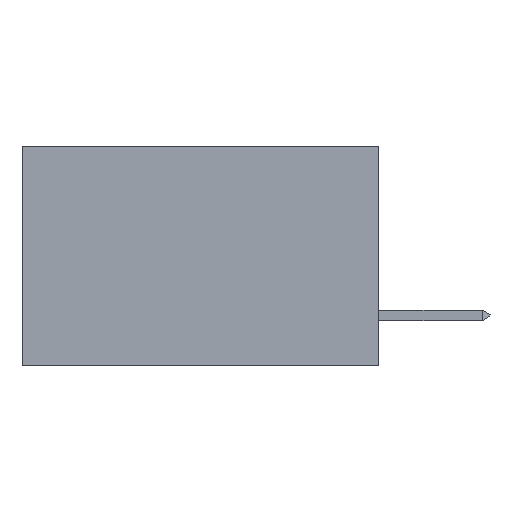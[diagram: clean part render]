
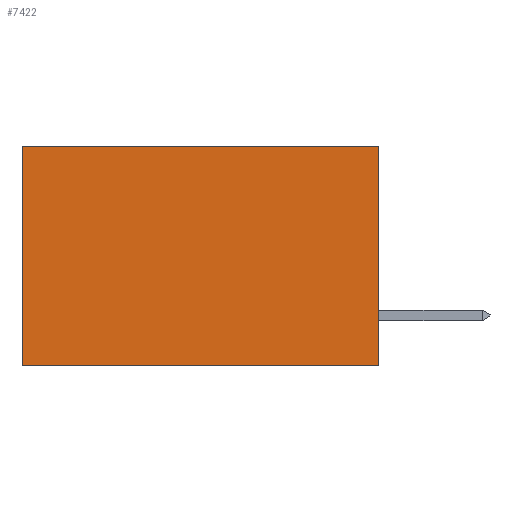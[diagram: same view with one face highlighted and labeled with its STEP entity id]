
A CAD part, left-side view. The second image highlights one B-rep face of the part: STEP entity #7422.
In plain terms, the highlighted planar face has unit normal (-1, 0, 0).
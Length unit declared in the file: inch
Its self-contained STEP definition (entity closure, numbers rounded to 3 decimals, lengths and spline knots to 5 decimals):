
#346 = EDGE_CURVE ( 'NONE', #3308, #4893, #1380, .T. ) ;
#358 = EDGE_CURVE ( 'NONE', #6321, #9454, #1969, .T. ) ;
#552 = AXIS2_PLACEMENT_3D ( 'NONE', #7037, #2612, #9248 ) ;
#845 = ORIENTED_EDGE ( 'NONE', *, *, #5354, .T. ) ;
#1380 = LINE ( 'NONE', #7633, #3596 ) ;
#1655 = DIRECTION ( 'NONE',  ( 0., 1., 0. ) ) ;
#1969 = LINE ( 'NONE', #5311, #6136 ) ;
#2228 = LINE ( 'NONE', #3424, #8669 ) ;
#2229 = CARTESIAN_POINT ( 'NONE',  ( 0.298, 0., -0.37 ) ) ;
#2612 = DIRECTION ( 'NONE',  ( 1., 0., 0. ) ) ;
#3308 = VERTEX_POINT ( 'NONE', #4462 ) ;
#3424 = CARTESIAN_POINT ( 'NONE',  ( 0.298, 0.6, 0. ) ) ;
#3534 = CARTESIAN_POINT ( 'NONE',  ( 0.298, 0.6, -0.37 ) ) ;
#3596 = VECTOR ( 'NONE', #5397, 39.37008 ) ;
#4080 = CARTESIAN_POINT ( 'NONE',  ( 0.298, 0.6, 0. ) ) ;
#4462 = CARTESIAN_POINT ( 'NONE',  ( 0.298, 0., 0. ) ) ;
#4559 = EDGE_CURVE ( 'NONE', #3308, #6321, #9398, .T. ) ;
#4621 = ORIENTED_EDGE ( 'NONE', *, *, #4559, .F. ) ;
#4893 = VERTEX_POINT ( 'NONE', #4080 ) ;
#5031 = VECTOR ( 'NONE', #8802, 39.37008 ) ;
#5099 = FACE_OUTER_BOUND ( 'NONE', #6977, .T. ) ;
#5311 = CARTESIAN_POINT ( 'NONE',  ( 0.298, 0., -0.37 ) ) ;
#5354 = EDGE_CURVE ( 'NONE', #4893, #9454, #2228, .T. ) ;
#5397 = DIRECTION ( 'NONE',  ( 0., 1., 0. ) ) ;
#6136 = VECTOR ( 'NONE', #1655, 39.37008 ) ;
#6321 = VERTEX_POINT ( 'NONE', #2229 ) ;
#6401 = DIRECTION ( 'NONE',  ( 0., 0., -1. ) ) ;
#6658 = CARTESIAN_POINT ( 'NONE',  ( 0.298, 0., 0. ) ) ;
#6977 = EDGE_LOOP ( 'NONE', ( #845, #9155, #4621, #7238 ) ) ;
#7005 = PLANE ( 'NONE',  #552 ) ;
#7037 = CARTESIAN_POINT ( 'NONE',  ( 0.298, 0., 0. ) ) ;
#7238 = ORIENTED_EDGE ( 'NONE', *, *, #346, .T. ) ;
#7422 = ADVANCED_FACE ( 'NONE', ( #5099 ), #7005, .F. ) ;
#7633 = CARTESIAN_POINT ( 'NONE',  ( 0.298, 0., 0. ) ) ;
#8669 = VECTOR ( 'NONE', #6401, 39.37008 ) ;
#8802 = DIRECTION ( 'NONE',  ( 0., 0., -1. ) ) ;
#9155 = ORIENTED_EDGE ( 'NONE', *, *, #358, .F. ) ;
#9248 = DIRECTION ( 'NONE',  ( 0., 0., -1. ) ) ;
#9398 = LINE ( 'NONE', #6658, #5031 ) ;
#9454 = VERTEX_POINT ( 'NONE', #3534 ) ;
